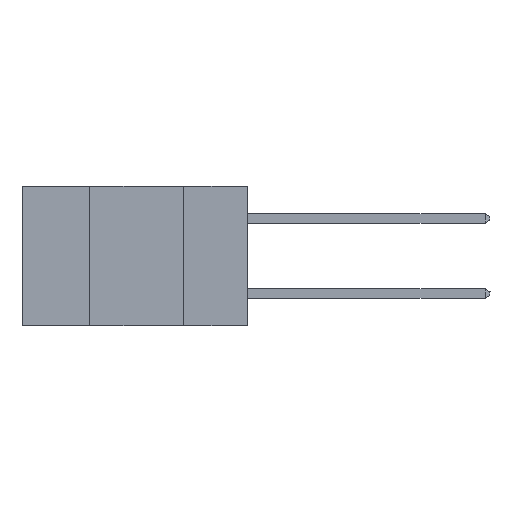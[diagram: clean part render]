
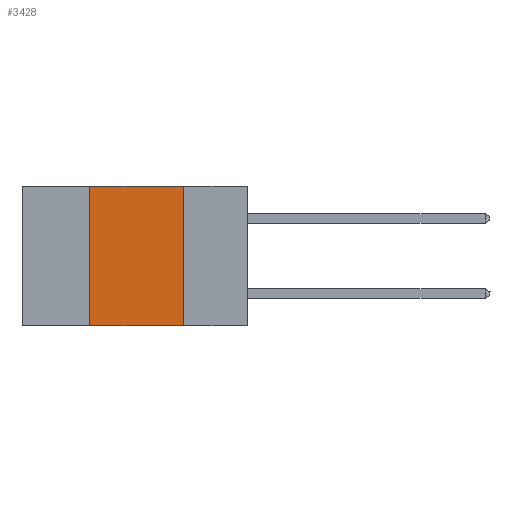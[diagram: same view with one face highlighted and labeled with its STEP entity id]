
A CAD part, left-side view. The second image highlights one B-rep face of the part: STEP entity #3428.
In plain terms, the highlighted planar face has unit normal (-1, 0, 0).
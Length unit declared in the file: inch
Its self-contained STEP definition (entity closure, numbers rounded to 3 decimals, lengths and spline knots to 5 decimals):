
#416 = EDGE_CURVE ( 'NONE', #13136, #23411, #24074, .T. ) ;
#627 = ORIENTED_EDGE ( 'NONE', *, *, #21022, .T. ) ;
#665 = CARTESIAN_POINT ( 'NONE',  ( 0., 0.42, -0.37 ) ) ;
#2831 = CARTESIAN_POINT ( 'NONE',  ( 0., 0.6, 0. ) ) ;
#3317 = VERTEX_POINT ( 'NONE', #665 ) ;
#3428 = ADVANCED_FACE ( 'NONE', ( #29877 ), #5812, .F. ) ;
#3770 = CARTESIAN_POINT ( 'NONE',  ( 0., 0.42, 0. ) ) ;
#4043 = DIRECTION ( 'NONE',  ( 0., -1., 0. ) ) ;
#4102 = VERTEX_POINT ( 'NONE', #22298 ) ;
#4337 = CARTESIAN_POINT ( 'NONE',  ( 0., 0.17, 0. ) ) ;
#4913 = VECTOR ( 'NONE', #5161, 39.37008 ) ;
#5161 = DIRECTION ( 'NONE',  ( 0., -1., 0. ) ) ;
#5812 = PLANE ( 'NONE',  #28554 ) ;
#6408 = ORIENTED_EDGE ( 'NONE', *, *, #19935, .F. ) ;
#7302 = EDGE_LOOP ( 'NONE', ( #16269, #6408, #27667, #627 ) ) ;
#12323 = VECTOR ( 'NONE', #21262, 39.37008 ) ;
#13116 = CARTESIAN_POINT ( 'NONE',  ( 0., 0.6, 0. ) ) ;
#13136 = VERTEX_POINT ( 'NONE', #25610 ) ;
#13557 = CARTESIAN_POINT ( 'NONE',  ( 0., 0.6, -0.37 ) ) ;
#15437 = DIRECTION ( 'NONE',  ( 0., 0., -1. ) ) ;
#16232 = VECTOR ( 'NONE', #27850, 39.37008 ) ;
#16269 = ORIENTED_EDGE ( 'NONE', *, *, #416, .F. ) ;
#18681 = CARTESIAN_POINT ( 'NONE',  ( 0., 0.17, -0.37 ) ) ;
#19935 = EDGE_CURVE ( 'NONE', #4102, #13136, #21956, .T. ) ;
#20188 = EDGE_CURVE ( 'NONE', #3317, #4102, #29563, .T. ) ;
#20696 = VECTOR ( 'NONE', #4043, 39.37008 ) ;
#21022 = EDGE_CURVE ( 'NONE', #3317, #23411, #28297, .T. ) ;
#21262 = DIRECTION ( 'NONE',  ( 0., 0., -1. ) ) ;
#21956 = LINE ( 'NONE', #2831, #4913 ) ;
#22298 = CARTESIAN_POINT ( 'NONE',  ( 0., 0.42, 0. ) ) ;
#23411 = VERTEX_POINT ( 'NONE', #18681 ) ;
#24074 = LINE ( 'NONE', #4337, #12323 ) ;
#25610 = CARTESIAN_POINT ( 'NONE',  ( 0., 0.17, 0. ) ) ;
#27667 = ORIENTED_EDGE ( 'NONE', *, *, #20188, .F. ) ;
#27850 = DIRECTION ( 'NONE',  ( 0., 0., 1. ) ) ;
#28297 = LINE ( 'NONE', #13557, #20696 ) ;
#28554 = AXIS2_PLACEMENT_3D ( 'NONE', #13116, #30004, #15437 ) ;
#29563 = LINE ( 'NONE', #3770, #16232 ) ;
#29877 = FACE_OUTER_BOUND ( 'NONE', #7302, .T. ) ;
#30004 = DIRECTION ( 'NONE',  ( 1., 0., 0. ) ) ;
